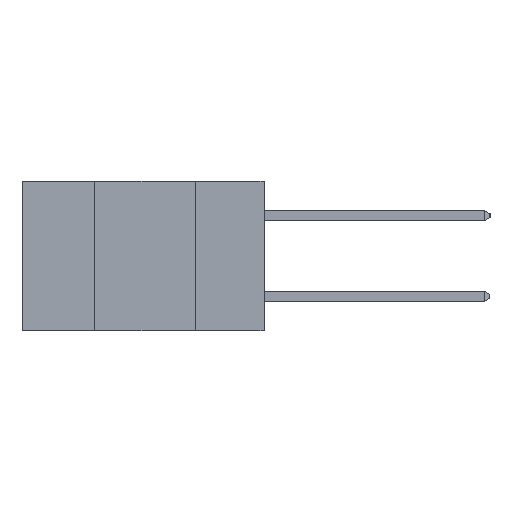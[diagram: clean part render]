
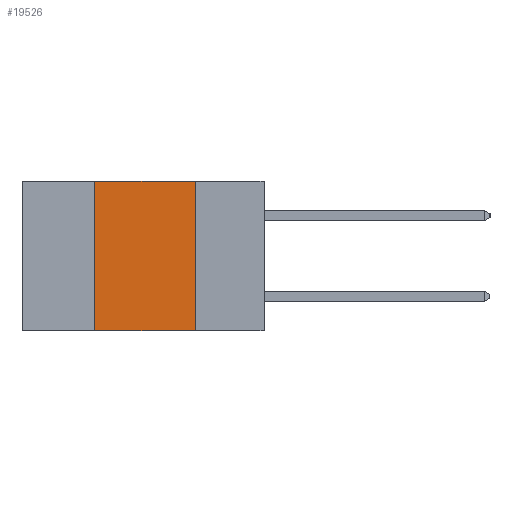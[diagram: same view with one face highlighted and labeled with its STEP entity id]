
A CAD part, left-side view. The second image highlights one B-rep face of the part: STEP entity #19526.
In plain terms, the highlighted planar face has unit normal (-1, 0, 0).
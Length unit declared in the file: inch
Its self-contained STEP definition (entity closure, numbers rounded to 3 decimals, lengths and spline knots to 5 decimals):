
#1052 = VECTOR ( 'NONE', #14362, 39.37008 ) ;
#1089 = CARTESIAN_POINT ( 'NONE',  ( 0., 0.17, -0.37 ) ) ;
#2293 = CARTESIAN_POINT ( 'NONE',  ( 0., 0.42, -0.37 ) ) ;
#2408 = DIRECTION ( 'NONE',  ( 0., 0., 1. ) ) ;
#3133 = CARTESIAN_POINT ( 'NONE',  ( 0., 0.6, 0. ) ) ;
#4260 = LINE ( 'NONE', #2293, #6738 ) ;
#6591 = DIRECTION ( 'NONE',  ( 1., 0., 0. ) ) ;
#6738 = VECTOR ( 'NONE', #2408, 39.37008 ) ;
#6985 = LINE ( 'NONE', #1089, #1052 ) ;
#8550 = EDGE_LOOP ( 'NONE', ( #11341, #20118, #17078, #9191 ) ) ;
#8605 = CARTESIAN_POINT ( 'NONE',  ( 0., 0.42, 0. ) ) ;
#8797 = PLANE ( 'NONE',  #13554 ) ;
#8835 = LINE ( 'NONE', #17928, #10857 ) ;
#9191 = ORIENTED_EDGE ( 'NONE', *, *, #15756, .T. ) ;
#10160 = LINE ( 'NONE', #13856, #15781 ) ;
#10474 = CARTESIAN_POINT ( 'NONE',  ( 0., 0.17, 0. ) ) ;
#10857 = VECTOR ( 'NONE', #23449, 39.37008 ) ;
#11061 = EDGE_CURVE ( 'NONE', #20324, #18738, #8835, .T. ) ;
#11063 = EDGE_CURVE ( 'NONE', #18738, #24023, #6985, .T. ) ;
#11341 = ORIENTED_EDGE ( 'NONE', *, *, #11063, .F. ) ;
#12543 = VERTEX_POINT ( 'NONE', #13238 ) ;
#13238 = CARTESIAN_POINT ( 'NONE',  ( 0., 0.42, -0.37 ) ) ;
#13554 = AXIS2_PLACEMENT_3D ( 'NONE', #3133, #6591, #15791 ) ;
#13856 = CARTESIAN_POINT ( 'NONE',  ( 0., 0.6, -0.37 ) ) ;
#14205 = CARTESIAN_POINT ( 'NONE',  ( 0., 0.17, -0.37 ) ) ;
#14323 = FACE_OUTER_BOUND ( 'NONE', #8550, .T. ) ;
#14362 = DIRECTION ( 'NONE',  ( 0., 0., -1. ) ) ;
#14443 = EDGE_CURVE ( 'NONE', #12543, #20324, #4260, .T. ) ;
#15756 = EDGE_CURVE ( 'NONE', #12543, #24023, #10160, .T. ) ;
#15781 = VECTOR ( 'NONE', #19141, 39.37008 ) ;
#15791 = DIRECTION ( 'NONE',  ( 0., 0., -1. ) ) ;
#17078 = ORIENTED_EDGE ( 'NONE', *, *, #14443, .F. ) ;
#17928 = CARTESIAN_POINT ( 'NONE',  ( 0., 0.6, 0. ) ) ;
#18738 = VERTEX_POINT ( 'NONE', #10474 ) ;
#19141 = DIRECTION ( 'NONE',  ( 0., -1., 0. ) ) ;
#19526 = ADVANCED_FACE ( 'NONE', ( #14323 ), #8797, .F. ) ;
#20118 = ORIENTED_EDGE ( 'NONE', *, *, #11061, .F. ) ;
#20324 = VERTEX_POINT ( 'NONE', #8605 ) ;
#23449 = DIRECTION ( 'NONE',  ( 0., -1., 0. ) ) ;
#24023 = VERTEX_POINT ( 'NONE', #14205 ) ;
